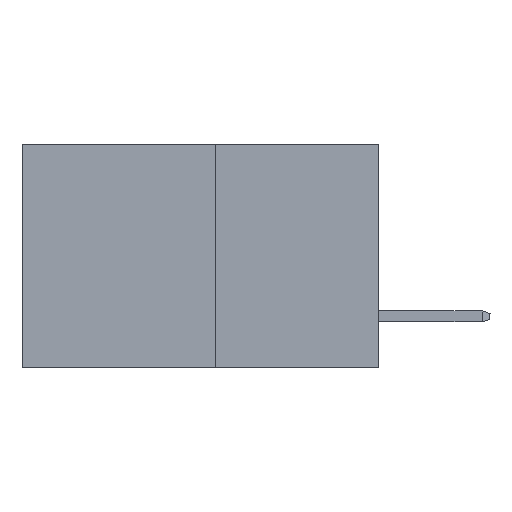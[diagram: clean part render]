
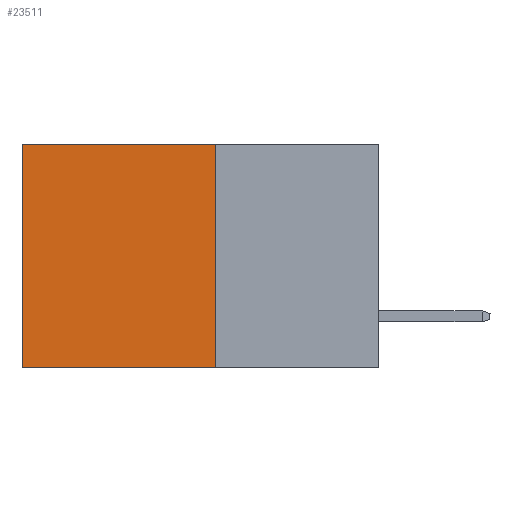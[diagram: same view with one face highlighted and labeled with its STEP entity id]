
A CAD part, left-side view. The second image highlights one B-rep face of the part: STEP entity #23511.
In plain terms, the highlighted planar face has unit normal (-1, 0, 0).
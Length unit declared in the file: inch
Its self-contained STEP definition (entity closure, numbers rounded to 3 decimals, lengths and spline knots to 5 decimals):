
#2281 = CARTESIAN_POINT ( 'NONE',  ( 0.277, 0.59, -0.37 ) ) ;
#2764 = CARTESIAN_POINT ( 'NONE',  ( 0.277, 0.27, -0.37 ) ) ;
#3362 = CARTESIAN_POINT ( 'NONE',  ( 0.277, 0.27, -0.37 ) ) ;
#3406 = CARTESIAN_POINT ( 'NONE',  ( 0.277, 0.59, 0. ) ) ;
#3763 = ORIENTED_EDGE ( 'NONE', *, *, #18963, .T. ) ;
#3777 = EDGE_CURVE ( 'NONE', #4315, #24745, #20778, .T. ) ;
#4190 = VECTOR ( 'NONE', #12081, 39.37008 ) ;
#4315 = VERTEX_POINT ( 'NONE', #19206 ) ;
#4718 = DIRECTION ( 'NONE',  ( 0., 0., -1. ) ) ;
#5846 = FACE_OUTER_BOUND ( 'NONE', #8503, .T. ) ;
#6178 = DIRECTION ( 'NONE',  ( 0., 1., 0. ) ) ;
#6598 = CARTESIAN_POINT ( 'NONE',  ( 0.277, 0.27, 0. ) ) ;
#6970 = ORIENTED_EDGE ( 'NONE', *, *, #23882, .F. ) ;
#7190 = PLANE ( 'NONE',  #19210 ) ;
#7224 = CARTESIAN_POINT ( 'NONE',  ( 0.277, 0.59, -0.37 ) ) ;
#7279 = DIRECTION ( 'NONE',  ( 0., 0., -1. ) ) ;
#8247 = VERTEX_POINT ( 'NONE', #3406 ) ;
#8503 = EDGE_LOOP ( 'NONE', ( #14135, #15116, #6970, #3763 ) ) ;
#9353 = LINE ( 'NONE', #2281, #4190 ) ;
#10353 = VERTEX_POINT ( 'NONE', #6598 ) ;
#12081 = DIRECTION ( 'NONE',  ( 0., 0., -1. ) ) ;
#12162 = LINE ( 'NONE', #2764, #21779 ) ;
#12723 = VECTOR ( 'NONE', #20613, 39.37008 ) ;
#14135 = ORIENTED_EDGE ( 'NONE', *, *, #14270, .T. ) ;
#14270 = EDGE_CURVE ( 'NONE', #8247, #24745, #9353, .T. ) ;
#15116 = ORIENTED_EDGE ( 'NONE', *, *, #3777, .F. ) ;
#15648 = VECTOR ( 'NONE', #6178, 39.37008 ) ;
#17807 = LINE ( 'NONE', #18663, #12723 ) ;
#18663 = CARTESIAN_POINT ( 'NONE',  ( 0.277, 0.27, 0. ) ) ;
#18788 = DIRECTION ( 'NONE',  ( 1., 0., 0. ) ) ;
#18963 = EDGE_CURVE ( 'NONE', #10353, #8247, #17807, .T. ) ;
#19206 = CARTESIAN_POINT ( 'NONE',  ( 0.277, 0.27, -0.37 ) ) ;
#19210 = AXIS2_PLACEMENT_3D ( 'NONE', #3362, #18788, #7279 ) ;
#20613 = DIRECTION ( 'NONE',  ( 0., 1., 0. ) ) ;
#20778 = LINE ( 'NONE', #21584, #15648 ) ;
#21584 = CARTESIAN_POINT ( 'NONE',  ( 0.277, 0.27, -0.37 ) ) ;
#21779 = VECTOR ( 'NONE', #4718, 39.37008 ) ;
#23511 = ADVANCED_FACE ( 'NONE', ( #5846 ), #7190, .F. ) ;
#23882 = EDGE_CURVE ( 'NONE', #10353, #4315, #12162, .T. ) ;
#24745 = VERTEX_POINT ( 'NONE', #7224 ) ;
